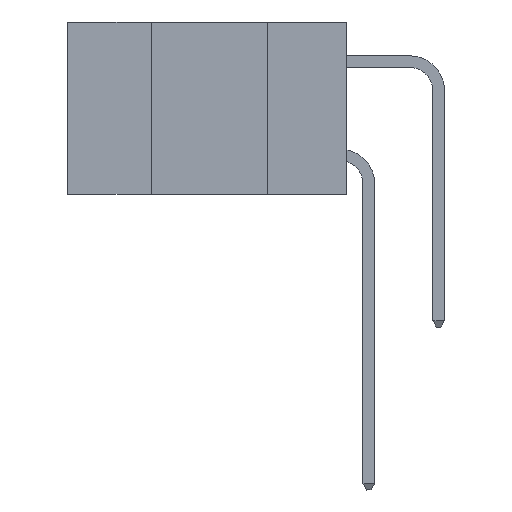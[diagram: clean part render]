
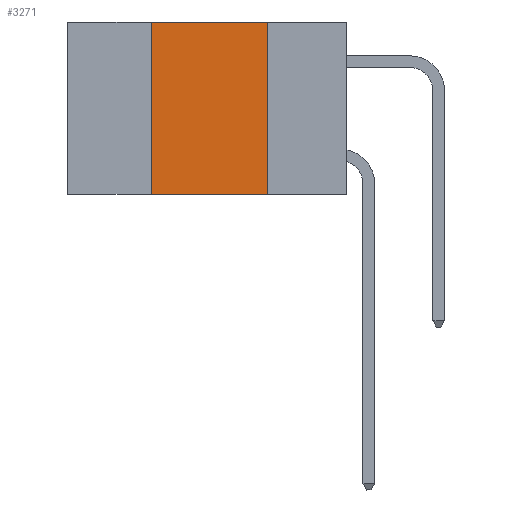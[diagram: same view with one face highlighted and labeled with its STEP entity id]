
A CAD part, left-side view. The second image highlights one B-rep face of the part: STEP entity #3271.
In plain terms, the highlighted planar face has unit normal (-1, 0, 0).
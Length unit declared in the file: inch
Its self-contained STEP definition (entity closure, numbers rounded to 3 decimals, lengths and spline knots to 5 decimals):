
#148 = EDGE_LOOP ( 'NONE', ( #683, #16982, #7323, #7838 ) ) ;
#419 = DIRECTION ( 'NONE',  ( 0., 0., -1. ) ) ;
#683 = ORIENTED_EDGE ( 'NONE', *, *, #15829, .F. ) ;
#1545 = EDGE_CURVE ( 'NONE', #4208, #5774, #1860, .T. ) ;
#1667 = VERTEX_POINT ( 'NONE', #18390 ) ;
#1860 = LINE ( 'NONE', #15084, #10109 ) ;
#3194 = CARTESIAN_POINT ( 'NONE',  ( 0., 0.17, 0. ) ) ;
#3271 = ADVANCED_FACE ( 'NONE', ( #14103 ), #8183, .F. ) ;
#4172 = CARTESIAN_POINT ( 'NONE',  ( 0., 0.42, 0. ) ) ;
#4208 = VERTEX_POINT ( 'NONE', #6524 ) ;
#4726 = VECTOR ( 'NONE', #9107, 39.37008 ) ;
#5680 = VERTEX_POINT ( 'NONE', #17781 ) ;
#5774 = VERTEX_POINT ( 'NONE', #13327 ) ;
#5859 = DIRECTION ( 'NONE',  ( 0., 0., -1. ) ) ;
#6326 = LINE ( 'NONE', #3194, #14968 ) ;
#6524 = CARTESIAN_POINT ( 'NONE',  ( 0., 0.42, -0.37 ) ) ;
#7094 = DIRECTION ( 'NONE',  ( 1., 0., 0. ) ) ;
#7323 = ORIENTED_EDGE ( 'NONE', *, *, #12612, .F. ) ;
#7838 = ORIENTED_EDGE ( 'NONE', *, *, #1545, .T. ) ;
#8183 = PLANE ( 'NONE',  #18026 ) ;
#9107 = DIRECTION ( 'NONE',  ( 0., -1., 0. ) ) ;
#10109 = VECTOR ( 'NONE', #15208, 39.37008 ) ;
#10891 = LINE ( 'NONE', #4172, #14235 ) ;
#11350 = CARTESIAN_POINT ( 'NONE',  ( 0., 0.6, 0. ) ) ;
#11648 = DIRECTION ( 'NONE',  ( 0., 0., 1. ) ) ;
#12612 = EDGE_CURVE ( 'NONE', #4208, #1667, #10891, .T. ) ;
#13327 = CARTESIAN_POINT ( 'NONE',  ( 0., 0.17, -0.37 ) ) ;
#14103 = FACE_OUTER_BOUND ( 'NONE', #148, .T. ) ;
#14235 = VECTOR ( 'NONE', #11648, 39.37008 ) ;
#14968 = VECTOR ( 'NONE', #419, 39.37008 ) ;
#15084 = CARTESIAN_POINT ( 'NONE',  ( 0., 0.6, -0.37 ) ) ;
#15208 = DIRECTION ( 'NONE',  ( 0., -1., 0. ) ) ;
#15224 = LINE ( 'NONE', #17509, #4726 ) ;
#15829 = EDGE_CURVE ( 'NONE', #5680, #5774, #6326, .T. ) ;
#16982 = ORIENTED_EDGE ( 'NONE', *, *, #18375, .F. ) ;
#17509 = CARTESIAN_POINT ( 'NONE',  ( 0., 0.6, 0. ) ) ;
#17781 = CARTESIAN_POINT ( 'NONE',  ( 0., 0.17, 0. ) ) ;
#18026 = AXIS2_PLACEMENT_3D ( 'NONE', #11350, #7094, #5859 ) ;
#18375 = EDGE_CURVE ( 'NONE', #1667, #5680, #15224, .T. ) ;
#18390 = CARTESIAN_POINT ( 'NONE',  ( 0., 0.42, 0. ) ) ;
